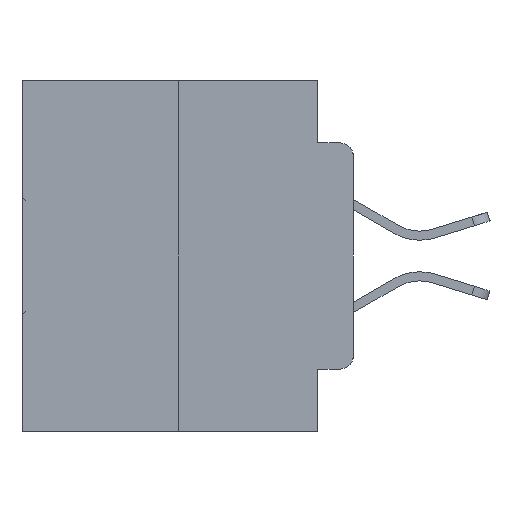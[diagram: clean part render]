
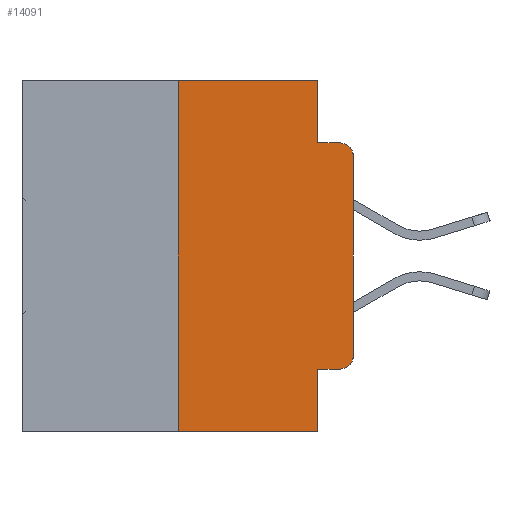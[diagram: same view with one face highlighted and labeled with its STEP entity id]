
A CAD part, left-side view. The second image highlights one B-rep face of the part: STEP entity #14091.
In plain terms, the highlighted planar face has unit normal (-1, 0, 0).
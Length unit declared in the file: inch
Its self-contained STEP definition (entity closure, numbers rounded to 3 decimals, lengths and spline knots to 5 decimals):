
#394 = VERTEX_POINT ( 'NONE', #22384 ) ;
#415 = VECTOR ( 'NONE', #26592, 39.37008 ) ;
#560 = AXIS2_PLACEMENT_3D ( 'NONE', #26651, #12152, #29059 ) ;
#760 = CARTESIAN_POINT ( 'NONE',  ( 0., 0.051, -0.0885 ) ) ;
#1126 = EDGE_CURVE ( 'NONE', #16148, #14832, #21913, .T. ) ;
#1150 = VECTOR ( 'NONE', #6539, 39.37008 ) ;
#1603 = ORIENTED_EDGE ( 'NONE', *, *, #30188, .T. ) ;
#1893 = EDGE_LOOP ( 'NONE', ( #12079, #24961, #7034, #13556, #19986, #15039, #21519, #3503, #1603, #8250 ) ) ;
#1901 = VERTEX_POINT ( 'NONE', #10081 ) ;
#2396 = DIRECTION ( 'NONE',  ( 0., 0., -1. ) ) ;
#3117 = VERTEX_POINT ( 'NONE', #760 ) ;
#3503 = ORIENTED_EDGE ( 'NONE', *, *, #19854, .F. ) ;
#4027 = CARTESIAN_POINT ( 'NONE',  ( 0., 0.25, 0. ) ) ;
#4809 = CARTESIAN_POINT ( 'NONE',  ( 0., 0.02, -0.3915 ) ) ;
#5489 = CIRCLE ( 'NONE', #10492, 0.02 ) ;
#5624 = VERTEX_POINT ( 'NONE', #6895 ) ;
#6003 = CARTESIAN_POINT ( 'NONE',  ( 0., 0.051, 0. ) ) ;
#6400 = VECTOR ( 'NONE', #2396, 39.37008 ) ;
#6539 = DIRECTION ( 'NONE',  ( 0., 0., 1. ) ) ;
#6789 = EDGE_CURVE ( 'NONE', #5624, #1901, #5489, .T. ) ;
#6834 = LINE ( 'NONE', #22229, #13372 ) ;
#6895 = CARTESIAN_POINT ( 'NONE',  ( 0., 0.02, -0.4115 ) ) ;
#7034 = ORIENTED_EDGE ( 'NONE', *, *, #31193, .F. ) ;
#7350 = VERTEX_POINT ( 'NONE', #20702 ) ;
#7459 = DIRECTION ( 'NONE',  ( 0., 0., -1. ) ) ;
#8250 = ORIENTED_EDGE ( 'NONE', *, *, #6789, .T. ) ;
#8346 = CARTESIAN_POINT ( 'NONE',  ( 0., 0.051, -0.4115 ) ) ;
#8591 = LINE ( 'NONE', #4027, #1150 ) ;
#8699 = CARTESIAN_POINT ( 'NONE',  ( 0., 0.473, -0.5 ) ) ;
#9508 = EDGE_CURVE ( 'NONE', #1901, #16148, #23235, .T. ) ;
#9593 = DIRECTION ( 'NONE',  ( 0., 0., -1. ) ) ;
#9654 = PLANE ( 'NONE',  #560 ) ;
#10081 = CARTESIAN_POINT ( 'NONE',  ( 0., 0., -0.3915 ) ) ;
#10492 = AXIS2_PLACEMENT_3D ( 'NONE', #4809, #24130, #9593 ) ;
#10841 = DIRECTION ( 'NONE',  ( 0., -1., 0. ) ) ;
#10869 = CARTESIAN_POINT ( 'NONE',  ( 0., 0.25, 0. ) ) ;
#11191 = DIRECTION ( 'NONE',  ( 0., -1., 0. ) ) ;
#11597 = LINE ( 'NONE', #6003, #24463 ) ;
#12079 = ORIENTED_EDGE ( 'NONE', *, *, #9508, .T. ) ;
#12134 = CARTESIAN_POINT ( 'NONE',  ( 0., 0.02, -0.1085 ) ) ;
#12152 = DIRECTION ( 'NONE',  ( 1., 0., 0. ) ) ;
#13265 = CARTESIAN_POINT ( 'NONE',  ( 0., 0., -0.1085 ) ) ;
#13372 = VECTOR ( 'NONE', #24678, 39.37008 ) ;
#13380 = EDGE_CURVE ( 'NONE', #25764, #394, #26554, .T. ) ;
#13556 = ORIENTED_EDGE ( 'NONE', *, *, #23147, .F. ) ;
#13836 = EDGE_CURVE ( 'NONE', #16635, #7350, #20025, .T. ) ;
#14091 = ADVANCED_FACE ( 'NONE', ( #25358 ), #9654, .F. ) ;
#14341 = VECTOR ( 'NONE', #11191, 39.37008 ) ;
#14832 = VERTEX_POINT ( 'NONE', #29415 ) ;
#15039 = ORIENTED_EDGE ( 'NONE', *, *, #21499, .F. ) ;
#15980 = VECTOR ( 'NONE', #30228, 39.37008 ) ;
#16148 = VERTEX_POINT ( 'NONE', #13265 ) ;
#16435 = LINE ( 'NONE', #8346, #22168 ) ;
#16635 = VERTEX_POINT ( 'NONE', #24695 ) ;
#19854 = EDGE_CURVE ( 'NONE', #29458, #7350, #25105, .T. ) ;
#19986 = ORIENTED_EDGE ( 'NONE', *, *, #13380, .F. ) ;
#20025 = LINE ( 'NONE', #8699, #14341 ) ;
#20702 = CARTESIAN_POINT ( 'NONE',  ( 0., 0.051, -0.5 ) ) ;
#21499 = EDGE_CURVE ( 'NONE', #16635, #25764, #8591, .T. ) ;
#21519 = ORIENTED_EDGE ( 'NONE', *, *, #13836, .T. ) ;
#21589 = CARTESIAN_POINT ( 'NONE',  ( 0., 0.473, 0. ) ) ;
#21913 = CIRCLE ( 'NONE', #24626, 0.02 ) ;
#22168 = VECTOR ( 'NONE', #10841, 39.37008 ) ;
#22229 = CARTESIAN_POINT ( 'NONE',  ( 0., 0.051, -0.0885 ) ) ;
#22384 = CARTESIAN_POINT ( 'NONE',  ( 0., 0.051, 0. ) ) ;
#23086 = DIRECTION ( 'NONE',  ( 0., 0., -1. ) ) ;
#23147 = EDGE_CURVE ( 'NONE', #394, #3117, #11597, .T. ) ;
#23235 = LINE ( 'NONE', #27849, #15980 ) ;
#24130 = DIRECTION ( 'NONE',  ( -1., 0., 0. ) ) ;
#24463 = VECTOR ( 'NONE', #23086, 39.37008 ) ;
#24626 = AXIS2_PLACEMENT_3D ( 'NONE', #12134, #29040, #7459 ) ;
#24678 = DIRECTION ( 'NONE',  ( 0., -1., 0. ) ) ;
#24695 = CARTESIAN_POINT ( 'NONE',  ( 0., 0.25, -0.5 ) ) ;
#24961 = ORIENTED_EDGE ( 'NONE', *, *, #1126, .T. ) ;
#25105 = LINE ( 'NONE', #31594, #6400 ) ;
#25358 = FACE_OUTER_BOUND ( 'NONE', #1893, .T. ) ;
#25764 = VERTEX_POINT ( 'NONE', #10869 ) ;
#26554 = LINE ( 'NONE', #21589, #415 ) ;
#26592 = DIRECTION ( 'NONE',  ( 0., -1., 0. ) ) ;
#26651 = CARTESIAN_POINT ( 'NONE',  ( 0., 0.473, 0. ) ) ;
#27205 = CARTESIAN_POINT ( 'NONE',  ( 0., 0.051, -0.4115 ) ) ;
#27849 = CARTESIAN_POINT ( 'NONE',  ( 0., 0., 0. ) ) ;
#29040 = DIRECTION ( 'NONE',  ( -1., 0., 0. ) ) ;
#29059 = DIRECTION ( 'NONE',  ( 0., 0., -1. ) ) ;
#29415 = CARTESIAN_POINT ( 'NONE',  ( 0., 0.02, -0.0885 ) ) ;
#29458 = VERTEX_POINT ( 'NONE', #27205 ) ;
#30188 = EDGE_CURVE ( 'NONE', #29458, #5624, #16435, .T. ) ;
#30228 = DIRECTION ( 'NONE',  ( 0., 0., 1. ) ) ;
#31193 = EDGE_CURVE ( 'NONE', #3117, #14832, #6834, .T. ) ;
#31594 = CARTESIAN_POINT ( 'NONE',  ( 0., 0.051, 0. ) ) ;
